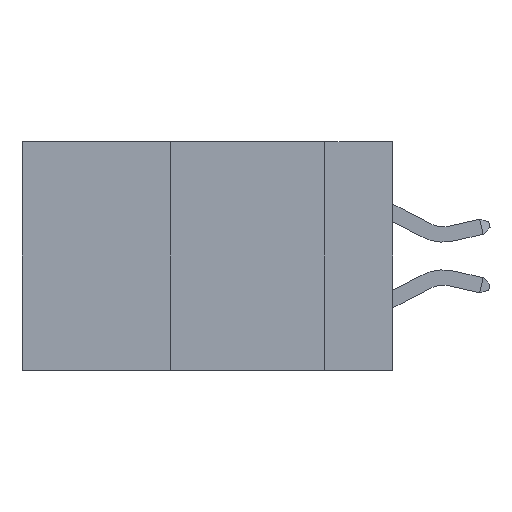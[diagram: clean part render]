
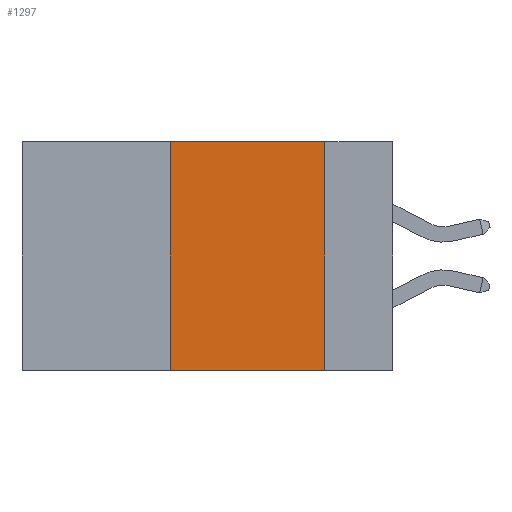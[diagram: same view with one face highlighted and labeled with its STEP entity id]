
A CAD part, left-side view. The second image highlights one B-rep face of the part: STEP entity #1297.
In plain terms, the highlighted planar face has unit normal (-1, 0, 0).
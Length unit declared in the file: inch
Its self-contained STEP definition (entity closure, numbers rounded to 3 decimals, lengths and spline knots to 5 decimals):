
#102 = ORIENTED_EDGE ( 'NONE', *, *, #817, .F. ) ;
#182 = CARTESIAN_POINT ( 'NONE',  ( 0., 0.6, 0. ) ) ;
#290 = CARTESIAN_POINT ( 'NONE',  ( 0., 0.11, 0. ) ) ;
#706 = CARTESIAN_POINT ( 'NONE',  ( 0., 0.6, 0. ) ) ;
#817 = EDGE_CURVE ( 'NONE', #5490, #6046, #10177, .T. ) ;
#969 = EDGE_CURVE ( 'NONE', #5490, #6741, #1043, .T. ) ;
#1043 = LINE ( 'NONE', #3034, #2701 ) ;
#1297 = ADVANCED_FACE ( 'NONE', ( #2696 ), #4712, .F. ) ;
#1519 = EDGE_CURVE ( 'NONE', #6046, #11156, #2975, .T. ) ;
#1560 = CARTESIAN_POINT ( 'NONE',  ( 0., 0.11, -0.37 ) ) ;
#1657 = DIRECTION ( 'NONE',  ( 1., 0., 0. ) ) ;
#2000 = ORIENTED_EDGE ( 'NONE', *, *, #1519, .F. ) ;
#2390 = EDGE_LOOP ( 'NONE', ( #11778, #2000, #102, #3722 ) ) ;
#2614 = AXIS2_PLACEMENT_3D ( 'NONE', #706, #1657, #8354 ) ;
#2696 = FACE_OUTER_BOUND ( 'NONE', #2390, .T. ) ;
#2701 = VECTOR ( 'NONE', #10678, 39.37008 ) ;
#2975 = LINE ( 'NONE', #182, #5486 ) ;
#3034 = CARTESIAN_POINT ( 'NONE',  ( 0., 0.6, -0.37 ) ) ;
#3722 = ORIENTED_EDGE ( 'NONE', *, *, #969, .T. ) ;
#4175 = DIRECTION ( 'NONE',  ( 0., -1., 0. ) ) ;
#4712 = PLANE ( 'NONE',  #2614 ) ;
#4773 = CARTESIAN_POINT ( 'NONE',  ( 0., 0.36, 0. ) ) ;
#5069 = VECTOR ( 'NONE', #7027, 39.37008 ) ;
#5486 = VECTOR ( 'NONE', #4175, 39.37008 ) ;
#5490 = VERTEX_POINT ( 'NONE', #5493 ) ;
#5493 = CARTESIAN_POINT ( 'NONE',  ( 0., 0.36, -0.37 ) ) ;
#5956 = VECTOR ( 'NONE', #8931, 39.37008 ) ;
#6046 = VERTEX_POINT ( 'NONE', #8699 ) ;
#6253 = LINE ( 'NONE', #11783, #5956 ) ;
#6741 = VERTEX_POINT ( 'NONE', #1560 ) ;
#7027 = DIRECTION ( 'NONE',  ( 0., 0., 1. ) ) ;
#8354 = DIRECTION ( 'NONE',  ( 0., 0., -1. ) ) ;
#8699 = CARTESIAN_POINT ( 'NONE',  ( 0., 0.36, 0. ) ) ;
#8931 = DIRECTION ( 'NONE',  ( 0., 0., -1. ) ) ;
#10177 = LINE ( 'NONE', #4773, #5069 ) ;
#10678 = DIRECTION ( 'NONE',  ( 0., -1., 0. ) ) ;
#11156 = VERTEX_POINT ( 'NONE', #290 ) ;
#11351 = EDGE_CURVE ( 'NONE', #11156, #6741, #6253, .T. ) ;
#11778 = ORIENTED_EDGE ( 'NONE', *, *, #11351, .F. ) ;
#11783 = CARTESIAN_POINT ( 'NONE',  ( 0., 0.11, 0. ) ) ;
